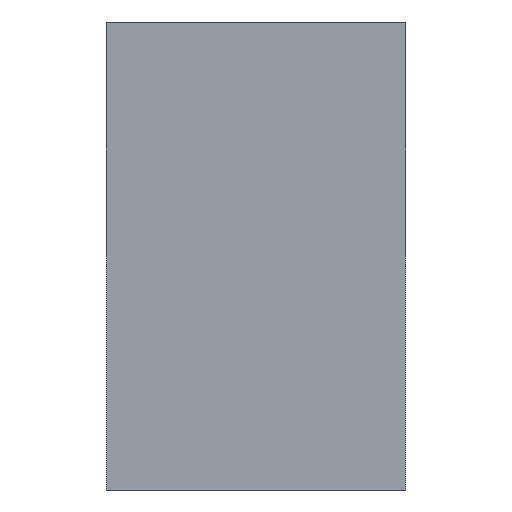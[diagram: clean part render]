
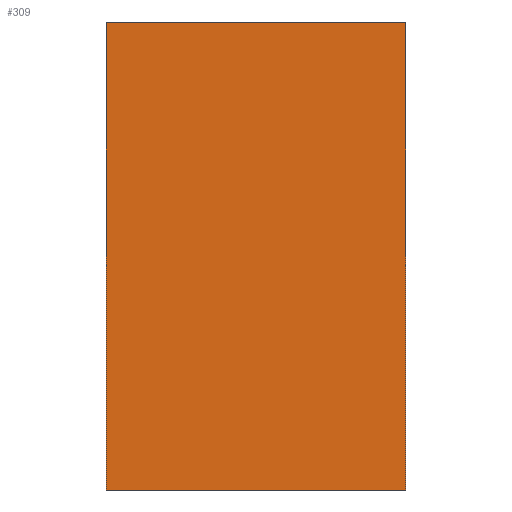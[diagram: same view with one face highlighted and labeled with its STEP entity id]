
A CAD part, front view. The second image highlights one B-rep face of the part: STEP entity #309.
In plain terms, the highlighted planar face has unit normal (0, -1, 0).
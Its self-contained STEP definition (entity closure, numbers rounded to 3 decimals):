
#3 = ORIENTED_EDGE ( 'NONE', *, *, #398, .T. ) ;
#12 = CARTESIAN_POINT ( 'NONE',  ( -4.644, -4.75, 2.5 ) ) ;
#38 = CARTESIAN_POINT ( 'NONE',  ( 4.644, -4.75, -12. ) ) ;
#39 = LINE ( 'NONE', #425, #56 ) ;
#50 = CARTESIAN_POINT ( 'NONE',  ( -4.644, -4.75, -12. ) ) ;
#55 = CARTESIAN_POINT ( 'NONE',  ( 4.644, -4.75, 2.5 ) ) ;
#56 = VECTOR ( 'NONE', #294, 1000. ) ;
#57 = EDGE_CURVE ( 'NONE', #226, #272, #39, .T. ) ;
#89 = EDGE_CURVE ( 'NONE', #272, #441, #237, .T. ) ;
#94 = VECTOR ( 'NONE', #428, 1000. ) ;
#162 = CARTESIAN_POINT ( 'NONE',  ( -4.644, -4.75, 2.5 ) ) ;
#182 = DIRECTION ( 'NONE',  ( 0., 0., -1. ) ) ;
#194 = AXIS2_PLACEMENT_3D ( 'NONE', #282, #281, #275 ) ;
#207 = CARTESIAN_POINT ( 'NONE',  ( -4.644, -4.75, 2.5 ) ) ;
#226 = VERTEX_POINT ( 'NONE', #38 ) ;
#237 = LINE ( 'NONE', #12, #94 ) ;
#264 = FACE_OUTER_BOUND ( 'NONE', #315, .T. ) ;
#272 = VERTEX_POINT ( 'NONE', #55 ) ;
#275 = DIRECTION ( 'NONE',  ( 0., 0., -1. ) ) ;
#281 = DIRECTION ( 'NONE',  ( 0., -1., 0. ) ) ;
#282 = CARTESIAN_POINT ( 'NONE',  ( 0., -4.75, 0. ) ) ;
#288 = PLANE ( 'NONE',  #194 ) ;
#294 = DIRECTION ( 'NONE',  ( 0., 0., 1. ) ) ;
#306 = DIRECTION ( 'NONE',  ( 1., 0., 0. ) ) ;
#309 = ADVANCED_FACE ( 'NONE', ( #264 ), #288, .T. ) ;
#315 = EDGE_LOOP ( 'NONE', ( #463, #3, #319, #388 ) ) ;
#319 = ORIENTED_EDGE ( 'NONE', *, *, #458, .T. ) ;
#388 = ORIENTED_EDGE ( 'NONE', *, *, #57, .T. ) ;
#398 = EDGE_CURVE ( 'NONE', #441, #478, #423, .T. ) ;
#401 = VECTOR ( 'NONE', #306, 1000. ) ;
#411 = LINE ( 'NONE', #50, #401 ) ;
#423 = LINE ( 'NONE', #207, #465 ) ;
#425 = CARTESIAN_POINT ( 'NONE',  ( 4.644, -4.75, 2.5 ) ) ;
#428 = DIRECTION ( 'NONE',  ( -1., 0., 0. ) ) ;
#441 = VERTEX_POINT ( 'NONE', #162 ) ;
#458 = EDGE_CURVE ( 'NONE', #478, #226, #411, .T. ) ;
#463 = ORIENTED_EDGE ( 'NONE', *, *, #89, .T. ) ;
#465 = VECTOR ( 'NONE', #182, 1000. ) ;
#466 = CARTESIAN_POINT ( 'NONE',  ( -4.644, -4.75, -12. ) ) ;
#478 = VERTEX_POINT ( 'NONE', #466 ) ;
